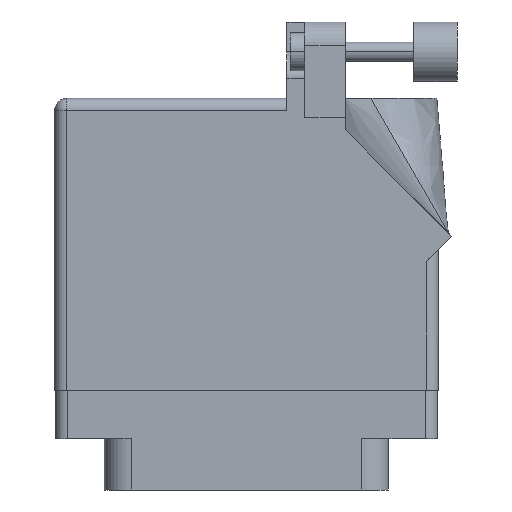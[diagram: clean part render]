
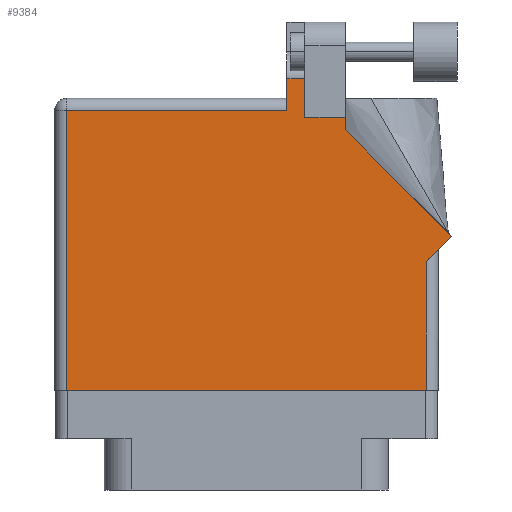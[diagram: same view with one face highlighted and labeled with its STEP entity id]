
A CAD part, front view. The second image highlights one B-rep face of the part: STEP entity #9384.
In plain terms, the highlighted face is planar.
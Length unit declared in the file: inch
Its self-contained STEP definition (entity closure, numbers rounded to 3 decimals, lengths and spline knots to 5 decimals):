
#605 = DIRECTION ( 'NONE',  ( -1., 0., 0. ) ) ;
#865 = EDGE_CURVE ( 'NONE', #21967, #17756, #26041, .T. ) ;
#984 = VECTOR ( 'NONE', #10312, 39.37008 ) ;
#2339 = VECTOR ( 'NONE', #2425, 39.37008 ) ;
#2425 = DIRECTION ( 'NONE',  ( 0., 1., 0. ) ) ;
#2567 = DIRECTION ( 'NONE',  ( 0., -1., 0. ) ) ;
#3048 = VERTEX_POINT ( 'NONE', #20298 ) ;
#3329 = VECTOR ( 'NONE', #2567, 39.37008 ) ;
#3621 = CARTESIAN_POINT ( 'NONE',  ( 1.07571, 0.70771, 0.455 ) ) ;
#3784 = VERTEX_POINT ( 'NONE', #35261 ) ;
#4157 = CARTESIAN_POINT ( 'NONE',  ( 0.943, 0.575, 0.455 ) ) ;
#4432 = LINE ( 'NONE', #5216, #14996 ) ;
#4505 = LINE ( 'NONE', #12797, #984 ) ;
#4632 = ORIENTED_EDGE ( 'NONE', *, *, #8875, .T. ) ;
#5216 = CARTESIAN_POINT ( 'NONE',  ( -0.943, -0.1, 0.455 ) ) ;
#5432 = DIRECTION ( 'NONE',  ( -1., 0., 0. ) ) ;
#5960 = VERTEX_POINT ( 'NONE', #22227 ) ;
#5969 = EDGE_CURVE ( 'NONE', #33167, #31074, #15137, .T. ) ;
#6381 = CARTESIAN_POINT ( 'NONE',  ( 0.519, 1.33, 0.455 ) ) ;
#7323 = CARTESIAN_POINT ( 'NONE',  ( -0.943, -0.1, 0.455 ) ) ;
#7922 = DIRECTION ( 'NONE',  ( -1., 0., 0. ) ) ;
#8394 = VECTOR ( 'NONE', #11612, 39.37008 ) ;
#8419 = VERTEX_POINT ( 'NONE', #31827 ) ;
#8875 = EDGE_CURVE ( 'NONE', #16240, #8419, #26652, .T. ) ;
#8889 = CARTESIAN_POINT ( 'NONE',  ( 1.005, 0.637, 0.455 ) ) ;
#9384 = ADVANCED_FACE ( 'NONE', ( #11603 ), #30731, .F. ) ;
#9834 = LINE ( 'NONE', #20410, #25296 ) ;
#9912 = ORIENTED_EDGE ( 'NONE', *, *, #20496, .T. ) ;
#10312 = DIRECTION ( 'NONE',  ( 0., 1., 0. ) ) ;
#10449 = ORIENTED_EDGE ( 'NONE', *, *, #25472, .T. ) ;
#10690 = AXIS2_PLACEMENT_3D ( 'NONE', #24804, #11108, #7922 ) ;
#10747 = LINE ( 'NONE', #3621, #20492 ) ;
#11108 = DIRECTION ( 'NONE',  ( 0., 0., -1. ) ) ;
#11603 = FACE_OUTER_BOUND ( 'NONE', #31349, .T. ) ;
#11612 = DIRECTION ( 'NONE',  ( 0.707, 0.707, 0. ) ) ;
#11633 = VECTOR ( 'NONE', #5432, 39.37008 ) ;
#12173 = ORIENTED_EDGE ( 'NONE', *, *, #24181, .T. ) ;
#12797 = CARTESIAN_POINT ( 'NONE',  ( 0.943, 0.637, 0.455 ) ) ;
#12837 = LINE ( 'NONE', #14743, #26526 ) ;
#13956 = CARTESIAN_POINT ( 'NONE',  ( 0.63677, 1.5315, 0.455 ) ) ;
#14032 = VERTEX_POINT ( 'NONE', #7323 ) ;
#14559 = VECTOR ( 'NONE', #36552, 39.37008 ) ;
#14743 = CARTESIAN_POINT ( 'NONE',  ( 0.519, 1.26442, 0.455 ) ) ;
#14996 = VECTOR ( 'NONE', #16691, 39.37008 ) ;
#15066 = VECTOR ( 'NONE', #605, 39.37008 ) ;
#15137 = LINE ( 'NONE', #24853, #2339 ) ;
#15248 = DIRECTION ( 'NONE',  ( 0., 1., 0. ) ) ;
#16024 = VERTEX_POINT ( 'NONE', #28930 ) ;
#16134 = CARTESIAN_POINT ( 'NONE',  ( 0.212, 1.43, 0.455 ) ) ;
#16240 = VERTEX_POINT ( 'NONE', #18677 ) ;
#16249 = ORIENTED_EDGE ( 'NONE', *, *, #17235, .T. ) ;
#16633 = DIRECTION ( 'NONE',  ( -0.707, 0.707, 0. ) ) ;
#16691 = DIRECTION ( 'NONE',  ( 0., -1., 0. ) ) ;
#17172 = EDGE_CURVE ( 'NONE', #3784, #33167, #21227, .T. ) ;
#17235 = EDGE_CURVE ( 'NONE', #5960, #3784, #12837, .T. ) ;
#17756 = VERTEX_POINT ( 'NONE', #20270 ) ;
#18677 = CARTESIAN_POINT ( 'NONE',  ( 0.212, 1.368, 0.455 ) ) ;
#20270 = CARTESIAN_POINT ( 'NONE',  ( 1.07571, 0.70771, 0.455 ) ) ;
#20298 = CARTESIAN_POINT ( 'NONE',  ( 0.212, 1.5315, 0.455 ) ) ;
#20410 = CARTESIAN_POINT ( 'NONE',  ( -1.005, -0.1, 0.455 ) ) ;
#20445 = EDGE_CURVE ( 'NONE', #8419, #14032, #4432, .T. ) ;
#20492 = VECTOR ( 'NONE', #16633, 39.37008 ) ;
#20496 = EDGE_CURVE ( 'NONE', #31074, #3048, #27824, .T. ) ;
#21227 = LINE ( 'NONE', #6381, #15066 ) ;
#21967 = VERTEX_POINT ( 'NONE', #4157 ) ;
#22227 = CARTESIAN_POINT ( 'NONE',  ( 0.519, 1.26442, 0.455 ) ) ;
#23465 = CARTESIAN_POINT ( 'NONE',  ( 0.306, 1.33, 0.455 ) ) ;
#23683 = ORIENTED_EDGE ( 'NONE', *, *, #36457, .T. ) ;
#24181 = EDGE_CURVE ( 'NONE', #17756, #5960, #10747, .T. ) ;
#24385 = ORIENTED_EDGE ( 'NONE', *, *, #865, .T. ) ;
#24804 = CARTESIAN_POINT ( 'NONE',  ( -1.005, 1.43, 0.455 ) ) ;
#24853 = CARTESIAN_POINT ( 'NONE',  ( 0.306, 1.33, 0.455 ) ) ;
#25296 = VECTOR ( 'NONE', #32122, 39.37008 ) ;
#25472 = EDGE_CURVE ( 'NONE', #16024, #21967, #4505, .T. ) ;
#26041 = LINE ( 'NONE', #8889, #8394 ) ;
#26526 = VECTOR ( 'NONE', #15248, 39.37008 ) ;
#26652 = LINE ( 'NONE', #36399, #11633 ) ;
#26842 = ORIENTED_EDGE ( 'NONE', *, *, #27593, .T. ) ;
#27155 = LINE ( 'NONE', #16134, #3329 ) ;
#27593 = EDGE_CURVE ( 'NONE', #14032, #16024, #9834, .T. ) ;
#27824 = LINE ( 'NONE', #13956, #14559 ) ;
#28930 = CARTESIAN_POINT ( 'NONE',  ( 0.943, -0.1, 0.455 ) ) ;
#29735 = ORIENTED_EDGE ( 'NONE', *, *, #20445, .T. ) ;
#30731 = PLANE ( 'NONE',  #10690 ) ;
#31074 = VERTEX_POINT ( 'NONE', #36210 ) ;
#31349 = EDGE_LOOP ( 'NONE', ( #35724, #9912, #23683, #4632, #29735, #26842, #10449, #24385, #12173, #16249, #32109 ) ) ;
#31827 = CARTESIAN_POINT ( 'NONE',  ( -0.943, 1.368, 0.455 ) ) ;
#32109 = ORIENTED_EDGE ( 'NONE', *, *, #17172, .T. ) ;
#32122 = DIRECTION ( 'NONE',  ( 1., 0., 0. ) ) ;
#33167 = VERTEX_POINT ( 'NONE', #23465 ) ;
#35261 = CARTESIAN_POINT ( 'NONE',  ( 0.519, 1.33, 0.455 ) ) ;
#35724 = ORIENTED_EDGE ( 'NONE', *, *, #5969, .T. ) ;
#36210 = CARTESIAN_POINT ( 'NONE',  ( 0.306, 1.5315, 0.455 ) ) ;
#36399 = CARTESIAN_POINT ( 'NONE',  ( -1.005, 1.368, 0.455 ) ) ;
#36457 = EDGE_CURVE ( 'NONE', #3048, #16240, #27155, .T. ) ;
#36552 = DIRECTION ( 'NONE',  ( -1., 0., 0. ) ) ;
